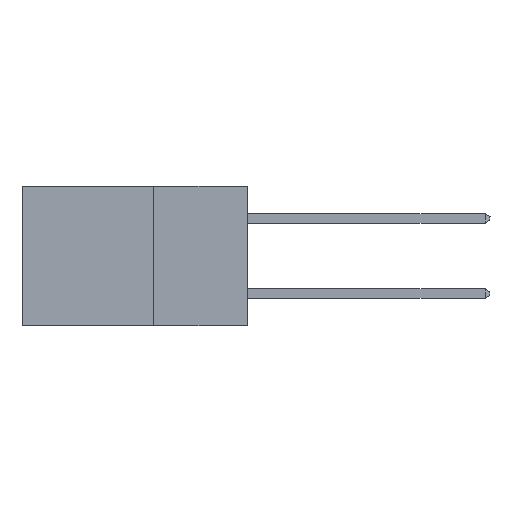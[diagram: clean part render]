
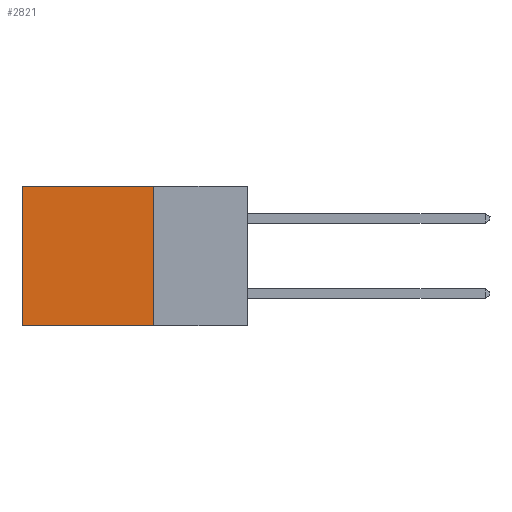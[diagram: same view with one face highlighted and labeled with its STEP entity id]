
A CAD part, left-side view. The second image highlights one B-rep face of the part: STEP entity #2821.
In plain terms, the highlighted planar face has unit normal (-1, 0, 0).
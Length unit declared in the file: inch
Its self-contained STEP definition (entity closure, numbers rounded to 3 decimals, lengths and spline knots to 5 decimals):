
#911 = VECTOR ( 'NONE', #4288, 39.37008 ) ;
#1997 = CARTESIAN_POINT ( 'NONE',  ( 0.2615, 0.6, 0. ) ) ;
#2248 = ORIENTED_EDGE ( 'NONE', *, *, #16722, .T. ) ;
#2475 = EDGE_CURVE ( 'NONE', #9058, #19043, #2581, .T. ) ;
#2581 = LINE ( 'NONE', #17253, #2808 ) ;
#2808 = VECTOR ( 'NONE', #17511, 39.37008 ) ;
#2821 = ADVANCED_FACE ( 'NONE', ( #11121 ), #7435, .F. ) ;
#4288 = DIRECTION ( 'NONE',  ( 0., 1., 0. ) ) ;
#6333 = CARTESIAN_POINT ( 'NONE',  ( 0.2615, 0.25, -0.37 ) ) ;
#6449 = LINE ( 'NONE', #6333, #911 ) ;
#6571 = EDGE_CURVE ( 'NONE', #18798, #17339, #12469, .T. ) ;
#7435 = PLANE ( 'NONE',  #18068 ) ;
#7615 = VECTOR ( 'NONE', #19778, 39.37008 ) ;
#9058 = VERTEX_POINT ( 'NONE', #1997 ) ;
#9288 = CARTESIAN_POINT ( 'NONE',  ( 0.2615, 0.6, -0.37 ) ) ;
#9637 = EDGE_LOOP ( 'NONE', ( #22707, #15611, #11439, #2248 ) ) ;
#9923 = CARTESIAN_POINT ( 'NONE',  ( 0.2615, 0.25, -0.37 ) ) ;
#11121 = FACE_OUTER_BOUND ( 'NONE', #9637, .T. ) ;
#11439 = ORIENTED_EDGE ( 'NONE', *, *, #6571, .F. ) ;
#12191 = LINE ( 'NONE', #19638, #7615 ) ;
#12469 = LINE ( 'NONE', #19561, #13500 ) ;
#13500 = VECTOR ( 'NONE', #23842, 39.37008 ) ;
#15409 = CARTESIAN_POINT ( 'NONE',  ( 0.2615, 0.25, 0. ) ) ;
#15611 = ORIENTED_EDGE ( 'NONE', *, *, #23036, .F. ) ;
#16722 = EDGE_CURVE ( 'NONE', #18798, #9058, #12191, .T. ) ;
#17253 = CARTESIAN_POINT ( 'NONE',  ( 0.2615, 0.6, -0.37 ) ) ;
#17339 = VERTEX_POINT ( 'NONE', #9923 ) ;
#17511 = DIRECTION ( 'NONE',  ( 0., 0., -1. ) ) ;
#18068 = AXIS2_PLACEMENT_3D ( 'NONE', #18355, #18466, #18227 ) ;
#18227 = DIRECTION ( 'NONE',  ( 0., 0., -1. ) ) ;
#18355 = CARTESIAN_POINT ( 'NONE',  ( 0.2615, 0.25, -0.37 ) ) ;
#18466 = DIRECTION ( 'NONE',  ( 1., 0., 0. ) ) ;
#18798 = VERTEX_POINT ( 'NONE', #15409 ) ;
#19043 = VERTEX_POINT ( 'NONE', #9288 ) ;
#19561 = CARTESIAN_POINT ( 'NONE',  ( 0.2615, 0.25, -0.37 ) ) ;
#19638 = CARTESIAN_POINT ( 'NONE',  ( 0.2615, 0.25, 0. ) ) ;
#19778 = DIRECTION ( 'NONE',  ( 0., 1., 0. ) ) ;
#22707 = ORIENTED_EDGE ( 'NONE', *, *, #2475, .T. ) ;
#23036 = EDGE_CURVE ( 'NONE', #17339, #19043, #6449, .T. ) ;
#23842 = DIRECTION ( 'NONE',  ( 0., 0., -1. ) ) ;
